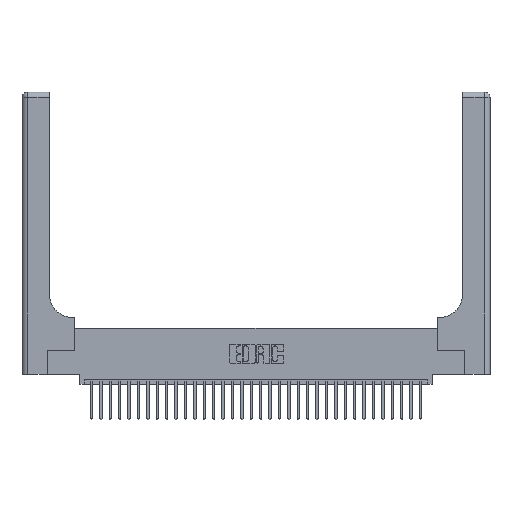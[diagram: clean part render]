
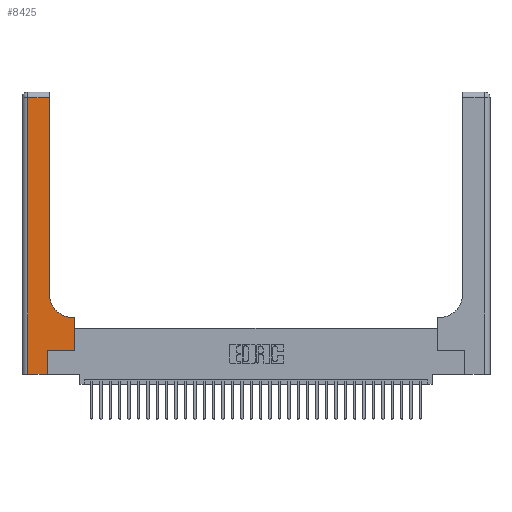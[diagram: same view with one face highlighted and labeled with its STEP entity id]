
A CAD part, top view. The second image highlights one B-rep face of the part: STEP entity #8425.
In plain terms, the highlighted planar face has unit normal (0, 0, 1).
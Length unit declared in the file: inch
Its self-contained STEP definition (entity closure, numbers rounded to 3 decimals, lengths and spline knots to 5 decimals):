
#269 = VERTEX_POINT ( 'NONE', #25953 ) ;
#317 = VERTEX_POINT ( 'NONE', #34154 ) ;
#713 = CARTESIAN_POINT ( 'NONE',  ( 0.06, 2.94, 0.37 ) ) ;
#804 = EDGE_CURVE ( 'NONE', #20306, #2366, #25096, .T. ) ;
#1415 = ORIENTED_EDGE ( 'NONE', *, *, #3402, .T. ) ;
#1897 = VECTOR ( 'NONE', #29547, 39.37008 ) ;
#2002 = VECTOR ( 'NONE', #10174, 39.37008 ) ;
#2074 = CARTESIAN_POINT ( 'NONE',  ( 0.5415, 0.85, 0.37 ) ) ;
#2366 = VERTEX_POINT ( 'NONE', #713 ) ;
#2461 = DIRECTION ( 'NONE',  ( 0., 1., 0. ) ) ;
#2507 = DIRECTION ( 'NONE',  ( 1., 0., 0. ) ) ;
#2951 = CARTESIAN_POINT ( 'NONE',  ( 0.2915, 0.6, 0.37 ) ) ;
#3402 = EDGE_CURVE ( 'NONE', #27424, #20306, #29861, .T. ) ;
#3876 = DIRECTION ( 'NONE',  ( 0., 1., 0. ) ) ;
#4693 = DIRECTION ( 'NONE',  ( 1., 0., 0. ) ) ;
#4814 = EDGE_LOOP ( 'NONE', ( #1415, #25754, #32102, #5989, #14716, #10233, #5748, #8103, #17753 ) ) ;
#4857 = VERTEX_POINT ( 'NONE', #10877 ) ;
#5748 = ORIENTED_EDGE ( 'NONE', *, *, #24442, .T. ) ;
#5900 = CARTESIAN_POINT ( 'NONE',  ( 0., 3., 0.37 ) ) ;
#5989 = ORIENTED_EDGE ( 'NONE', *, *, #12023, .T. ) ;
#6275 = EDGE_CURVE ( 'NONE', #269, #4857, #9768, .T. ) ;
#7849 = CARTESIAN_POINT ( 'NONE',  ( 0.2915, 2.94, 0.37 ) ) ;
#8103 = ORIENTED_EDGE ( 'NONE', *, *, #15636, .T. ) ;
#8425 = ADVANCED_FACE ( 'NONE', ( #24272 ), #27229, .F. ) ;
#8519 = AXIS2_PLACEMENT_3D ( 'NONE', #2074, #20622, #4693 ) ;
#8781 = VERTEX_POINT ( 'NONE', #23486 ) ;
#8991 = LINE ( 'NONE', #20776, #2002 ) ;
#9333 = CARTESIAN_POINT ( 'NONE',  ( 0., 2.94, 0.37 ) ) ;
#9768 = LINE ( 'NONE', #17080, #16029 ) ;
#10174 = DIRECTION ( 'NONE',  ( 0., -1., 0. ) ) ;
#10233 = ORIENTED_EDGE ( 'NONE', *, *, #34291, .T. ) ;
#10277 = CARTESIAN_POINT ( 'NONE',  ( 0., 0., 0.37 ) ) ;
#10877 = CARTESIAN_POINT ( 'NONE',  ( 0.269, 0.25, 0.37 ) ) ;
#11230 = DIRECTION ( 'NONE',  ( 0., 0., -1. ) ) ;
#11261 = VERTEX_POINT ( 'NONE', #31148 ) ;
#11481 = VECTOR ( 'NONE', #2507, 39.37008 ) ;
#11716 = VECTOR ( 'NONE', #28016, 39.37008 ) ;
#12022 = VERTEX_POINT ( 'NONE', #28927 ) ;
#12023 = EDGE_CURVE ( 'NONE', #11261, #269, #25322, .T. ) ;
#14716 = ORIENTED_EDGE ( 'NONE', *, *, #6275, .T. ) ;
#15636 = EDGE_CURVE ( 'NONE', #317, #12022, #15982, .T. ) ;
#15982 = LINE ( 'NONE', #2951, #1897 ) ;
#16029 = VECTOR ( 'NONE', #3876, 39.37008 ) ;
#16046 = CIRCLE ( 'NONE', #8519, 0.25 ) ;
#17080 = CARTESIAN_POINT ( 'NONE',  ( 0.269, 0., 0.37 ) ) ;
#17753 = ORIENTED_EDGE ( 'NONE', *, *, #33662, .T. ) ;
#18188 = VECTOR ( 'NONE', #34236, 39.37008 ) ;
#18376 = CARTESIAN_POINT ( 'NONE',  ( 0.269, 0.25, 0.37 ) ) ;
#19443 = VECTOR ( 'NONE', #2461, 39.37008 ) ;
#20306 = VERTEX_POINT ( 'NONE', #7849 ) ;
#20622 = DIRECTION ( 'NONE',  ( 0., 0., -1. ) ) ;
#20776 = CARTESIAN_POINT ( 'NONE',  ( 0.06, 3., 0.37 ) ) ;
#21315 = CARTESIAN_POINT ( 'NONE',  ( 0.2915, 3., 0.37 ) ) ;
#22216 = CARTESIAN_POINT ( 'NONE',  ( 0.2915, 0.85, 0.37 ) ) ;
#22827 = VECTOR ( 'NONE', #31889, 39.37008 ) ;
#23486 = CARTESIAN_POINT ( 'NONE',  ( 0.5585, 0.25, 0.37 ) ) ;
#24272 = FACE_OUTER_BOUND ( 'NONE', #4814, .T. ) ;
#24442 = EDGE_CURVE ( 'NONE', #8781, #317, #26555, .T. ) ;
#25096 = LINE ( 'NONE', #9333, #11716 ) ;
#25322 = LINE ( 'NONE', #10277, #18188 ) ;
#25754 = ORIENTED_EDGE ( 'NONE', *, *, #804, .T. ) ;
#25875 = EDGE_CURVE ( 'NONE', #2366, #11261, #8991, .T. ) ;
#25953 = CARTESIAN_POINT ( 'NONE',  ( 0.269, 0., 0.37 ) ) ;
#26502 = CARTESIAN_POINT ( 'NONE',  ( 0.5585, 0.25, 0.37 ) ) ;
#26555 = LINE ( 'NONE', #26502, #19443 ) ;
#27229 = PLANE ( 'NONE',  #30983 ) ;
#27424 = VERTEX_POINT ( 'NONE', #22216 ) ;
#28016 = DIRECTION ( 'NONE',  ( -1., 0., 0. ) ) ;
#28927 = CARTESIAN_POINT ( 'NONE',  ( 0.5415, 0.6, 0.37 ) ) ;
#29547 = DIRECTION ( 'NONE',  ( -1., 0., 0. ) ) ;
#29861 = LINE ( 'NONE', #21315, #22827 ) ;
#29871 = DIRECTION ( 'NONE',  ( -1., 0., 0. ) ) ;
#30983 = AXIS2_PLACEMENT_3D ( 'NONE', #5900, #11230, #29871 ) ;
#31148 = CARTESIAN_POINT ( 'NONE',  ( 0.06, 0., 0.37 ) ) ;
#31881 = LINE ( 'NONE', #18376, #11481 ) ;
#31889 = DIRECTION ( 'NONE',  ( 0., 1., 0. ) ) ;
#32102 = ORIENTED_EDGE ( 'NONE', *, *, #25875, .T. ) ;
#33662 = EDGE_CURVE ( 'NONE', #12022, #27424, #16046, .T. ) ;
#34154 = CARTESIAN_POINT ( 'NONE',  ( 0.5585, 0.6, 0.37 ) ) ;
#34236 = DIRECTION ( 'NONE',  ( 1., 0., 0. ) ) ;
#34291 = EDGE_CURVE ( 'NONE', #4857, #8781, #31881, .T. ) ;
